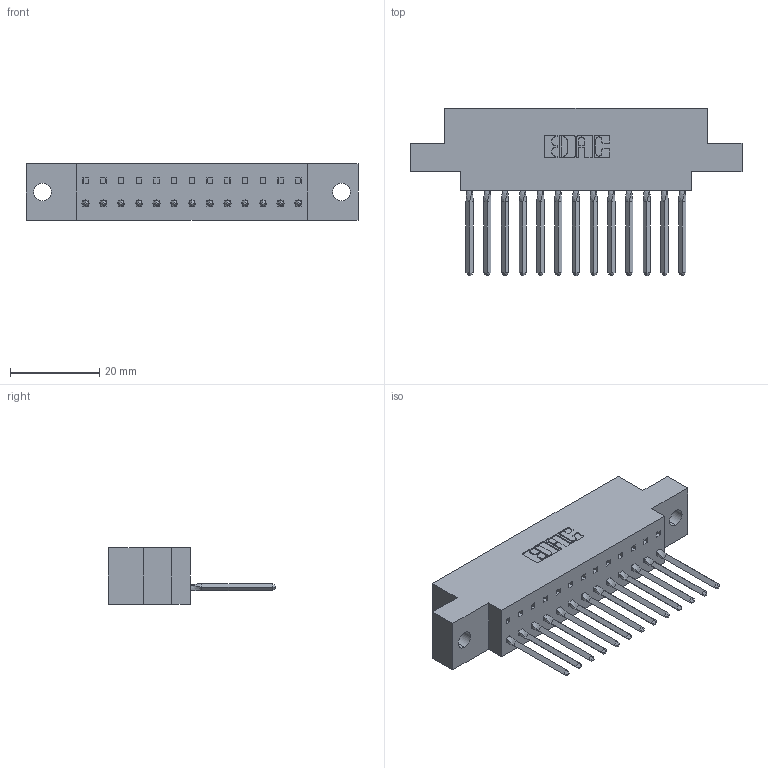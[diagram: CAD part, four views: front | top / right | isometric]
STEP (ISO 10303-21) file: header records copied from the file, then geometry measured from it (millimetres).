
FILE_DESCRIPTION (( 'STEP AP203' ), '1' );
FILE_NAME ('317-013-541-604.STEP', '2020-02-27T14:26:24', ( '' ), ( '' ), 'SwSTEP 2.0', 'SolidWorks 2016', '' );
FILE_SCHEMA (( 'CONFIG_CONTROL_DESIGN' ));
Length unit declared in the file: inch
Products named in the file (3): 317 Part_.156 Dia - TH; 317-290-002_541; 317-013-541-604
Assembly tree (14 placements, depth 2):
  317-013-541-604
    317 Part_.156 Dia - TH
    317-290-002_541  x13
Bounding box: 74.22 x 37.34 x 12.7 mm (x, y, z)
Volume: 11056.2 mm3; surface area: 14474.3 mm2
Topology: 14 solids, 14 shells, 2078 faces, 5917 edges, 3848 vertices
Faces by surface type: plane 1670, cylinder 356, bspline 52
Entity records: 23972 total; most frequent: CARTESIAN_POINT 4888, ORIENTED_EDGE 4154, DIRECTION 3391, EDGE_CURVE 2077, VECTOR 1713, LINE 1713, VERTEX_POINT 1376, AXIS2_PLACEMENT_3D 839
